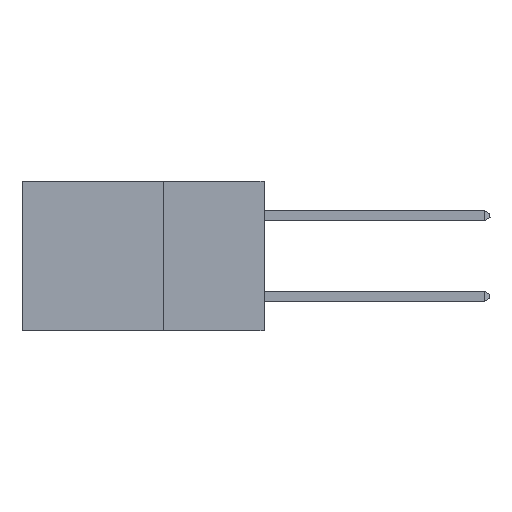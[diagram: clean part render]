
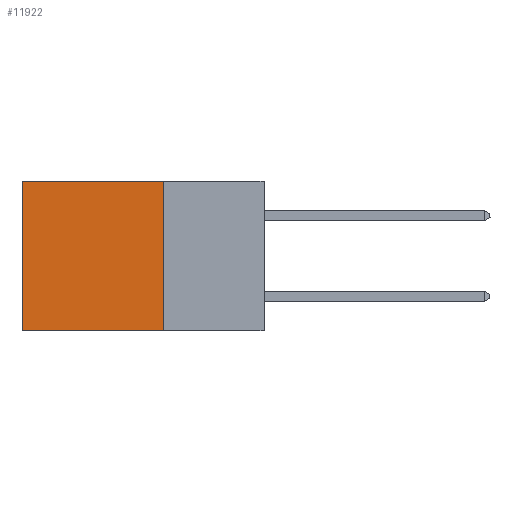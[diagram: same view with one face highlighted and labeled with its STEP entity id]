
A CAD part, left-side view. The second image highlights one B-rep face of the part: STEP entity #11922.
In plain terms, the highlighted planar face has unit normal (-1, 0, 0).
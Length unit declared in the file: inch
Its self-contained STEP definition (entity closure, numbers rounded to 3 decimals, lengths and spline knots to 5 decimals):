
#273 = VERTEX_POINT ( 'NONE', #3115 ) ;
#588 = ORIENTED_EDGE ( 'NONE', *, *, #14874, .F. ) ;
#1533 = EDGE_CURVE ( 'NONE', #17091, #15472, #12120, .T. ) ;
#2105 = CARTESIAN_POINT ( 'NONE',  ( 0.298, 0.25, -0.37 ) ) ;
#2184 = DIRECTION ( 'NONE',  ( 0., 0., -1. ) ) ;
#2498 = CARTESIAN_POINT ( 'NONE',  ( 0.298, 0.25, 0. ) ) ;
#3115 = CARTESIAN_POINT ( 'NONE',  ( 0.298, 0.25, 0. ) ) ;
#3744 = CARTESIAN_POINT ( 'NONE',  ( 0.298, 0.6, 0. ) ) ;
#5935 = VERTEX_POINT ( 'NONE', #2105 ) ;
#6005 = EDGE_CURVE ( 'NONE', #5935, #15472, #15299, .T. ) ;
#6159 = AXIS2_PLACEMENT_3D ( 'NONE', #14801, #7082, #8585 ) ;
#7082 = DIRECTION ( 'NONE',  ( 1., 0., 0. ) ) ;
#8096 = VECTOR ( 'NONE', #2184, 39.37008 ) ;
#8585 = DIRECTION ( 'NONE',  ( 0., 0., -1. ) ) ;
#8756 = FACE_OUTER_BOUND ( 'NONE', #10920, .T. ) ;
#10920 = EDGE_LOOP ( 'NONE', ( #19211, #19496, #588, #14610 ) ) ;
#11281 = VECTOR ( 'NONE', #12325, 39.37008 ) ;
#11922 = ADVANCED_FACE ( 'NONE', ( #8756 ), #19309, .F. ) ;
#12120 = LINE ( 'NONE', #14247, #8096 ) ;
#12179 = LINE ( 'NONE', #15795, #19041 ) ;
#12325 = DIRECTION ( 'NONE',  ( 0., 1., 0. ) ) ;
#12598 = EDGE_CURVE ( 'NONE', #273, #17091, #18206, .T. ) ;
#12710 = CARTESIAN_POINT ( 'NONE',  ( 0.298, 0.25, -0.37 ) ) ;
#13164 = DIRECTION ( 'NONE',  ( 0., 1., 0. ) ) ;
#13445 = VECTOR ( 'NONE', #13164, 39.37008 ) ;
#14247 = CARTESIAN_POINT ( 'NONE',  ( 0.298, 0.6, 0. ) ) ;
#14610 = ORIENTED_EDGE ( 'NONE', *, *, #12598, .T. ) ;
#14801 = CARTESIAN_POINT ( 'NONE',  ( 0.298, 0.25, 0. ) ) ;
#14874 = EDGE_CURVE ( 'NONE', #273, #5935, #12179, .T. ) ;
#15299 = LINE ( 'NONE', #12710, #11281 ) ;
#15472 = VERTEX_POINT ( 'NONE', #19376 ) ;
#15590 = DIRECTION ( 'NONE',  ( 0., 0., -1. ) ) ;
#15795 = CARTESIAN_POINT ( 'NONE',  ( 0.298, 0.25, 0. ) ) ;
#17091 = VERTEX_POINT ( 'NONE', #3744 ) ;
#18206 = LINE ( 'NONE', #2498, #13445 ) ;
#19041 = VECTOR ( 'NONE', #15590, 39.37008 ) ;
#19211 = ORIENTED_EDGE ( 'NONE', *, *, #1533, .T. ) ;
#19309 = PLANE ( 'NONE',  #6159 ) ;
#19376 = CARTESIAN_POINT ( 'NONE',  ( 0.298, 0.6, -0.37 ) ) ;
#19496 = ORIENTED_EDGE ( 'NONE', *, *, #6005, .F. ) ;
